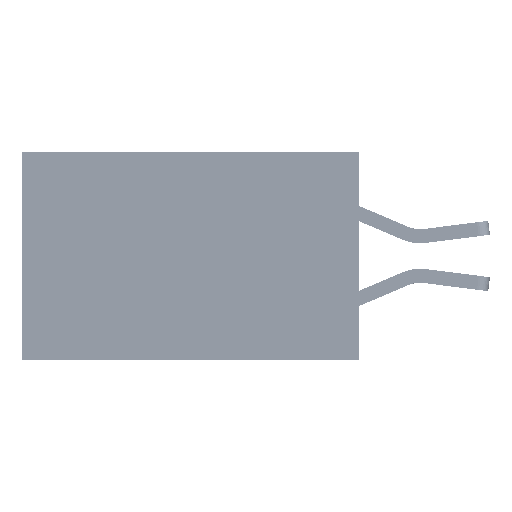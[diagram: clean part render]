
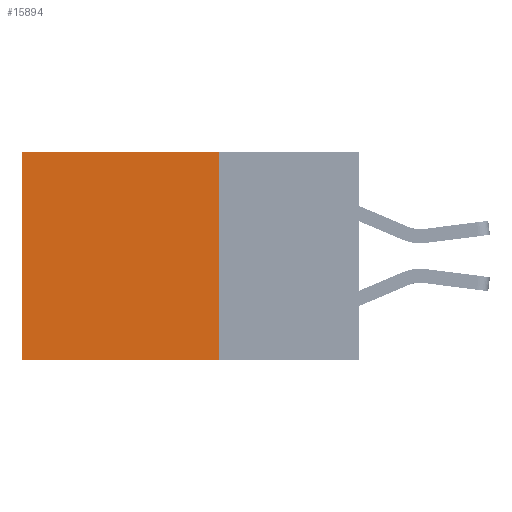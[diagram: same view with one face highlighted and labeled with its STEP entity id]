
A CAD part, left-side view. The second image highlights one B-rep face of the part: STEP entity #15894.
In plain terms, the highlighted planar face has unit normal (-1, 0, 0).
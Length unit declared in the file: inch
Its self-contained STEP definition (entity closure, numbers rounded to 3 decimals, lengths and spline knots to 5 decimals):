
#1164 = CARTESIAN_POINT ( 'NONE',  ( 0.2875, 0.6, 0. ) ) ;
#1776 = FACE_OUTER_BOUND ( 'NONE', #10597, .T. ) ;
#4926 = VERTEX_POINT ( 'NONE', #27900 ) ;
#8152 = DIRECTION ( 'NONE',  ( 0., 0., -1. ) ) ;
#10597 = EDGE_LOOP ( 'NONE', ( #27642, #19178, #15802, #28197 ) ) ;
#11056 = CARTESIAN_POINT ( 'NONE',  ( 0.2875, 0.25, 0. ) ) ;
#14160 = VECTOR ( 'NONE', #19133, 39.37008 ) ;
#14577 = DIRECTION ( 'NONE',  ( 0., 1., 0. ) ) ;
#14946 = VECTOR ( 'NONE', #34387, 39.37008 ) ;
#15802 = ORIENTED_EDGE ( 'NONE', *, *, #39621, .F. ) ;
#15894 = ADVANCED_FACE ( 'NONE', ( #1776 ), #33245, .F. ) ;
#16237 = VERTEX_POINT ( 'NONE', #18107 ) ;
#17074 = CARTESIAN_POINT ( 'NONE',  ( 0.2875, 0.6, -0.37 ) ) ;
#18107 = CARTESIAN_POINT ( 'NONE',  ( 0.2875, 0.25, -0.37 ) ) ;
#19133 = DIRECTION ( 'NONE',  ( 0., 0., -1. ) ) ;
#19178 = ORIENTED_EDGE ( 'NONE', *, *, #28450, .F. ) ;
#19394 = DIRECTION ( 'NONE',  ( 1., 0., 0. ) ) ;
#22559 = CARTESIAN_POINT ( 'NONE',  ( 0.2875, 0.25, 0. ) ) ;
#24469 = AXIS2_PLACEMENT_3D ( 'NONE', #40219, #19394, #43670 ) ;
#24551 = LINE ( 'NONE', #22559, #14160 ) ;
#27407 = LINE ( 'NONE', #1164, #44752 ) ;
#27642 = ORIENTED_EDGE ( 'NONE', *, *, #38026, .T. ) ;
#27900 = CARTESIAN_POINT ( 'NONE',  ( 0.2875, 0.6, 0. ) ) ;
#28197 = ORIENTED_EDGE ( 'NONE', *, *, #35605, .T. ) ;
#28450 = EDGE_CURVE ( 'NONE', #16237, #32824, #33509, .T. ) ;
#29101 = CARTESIAN_POINT ( 'NONE',  ( 0.2875, 0.25, 0. ) ) ;
#30868 = CARTESIAN_POINT ( 'NONE',  ( 0.2875, 0.25, -0.37 ) ) ;
#32824 = VERTEX_POINT ( 'NONE', #17074 ) ;
#33177 = VERTEX_POINT ( 'NONE', #29101 ) ;
#33245 = PLANE ( 'NONE',  #24469 ) ;
#33509 = LINE ( 'NONE', #30868, #14946 ) ;
#34387 = DIRECTION ( 'NONE',  ( 0., 1., 0. ) ) ;
#35605 = EDGE_CURVE ( 'NONE', #33177, #4926, #44904, .T. ) ;
#38026 = EDGE_CURVE ( 'NONE', #4926, #32824, #27407, .T. ) ;
#39621 = EDGE_CURVE ( 'NONE', #33177, #16237, #24551, .T. ) ;
#40219 = CARTESIAN_POINT ( 'NONE',  ( 0.2875, 0.25, 0. ) ) ;
#43670 = DIRECTION ( 'NONE',  ( 0., 0., -1. ) ) ;
#43857 = VECTOR ( 'NONE', #14577, 39.37008 ) ;
#44752 = VECTOR ( 'NONE', #8152, 39.37008 ) ;
#44904 = LINE ( 'NONE', #11056, #43857 ) ;
